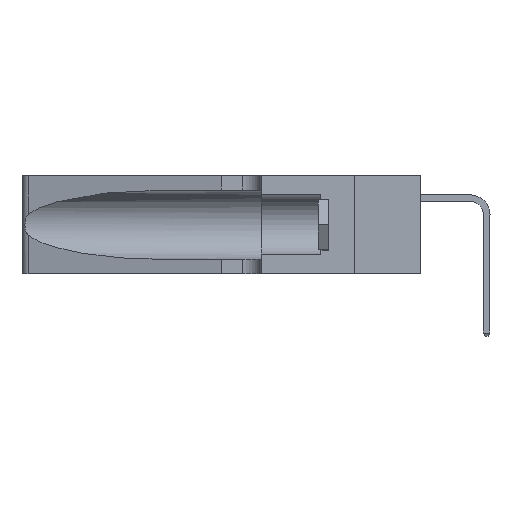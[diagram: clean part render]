
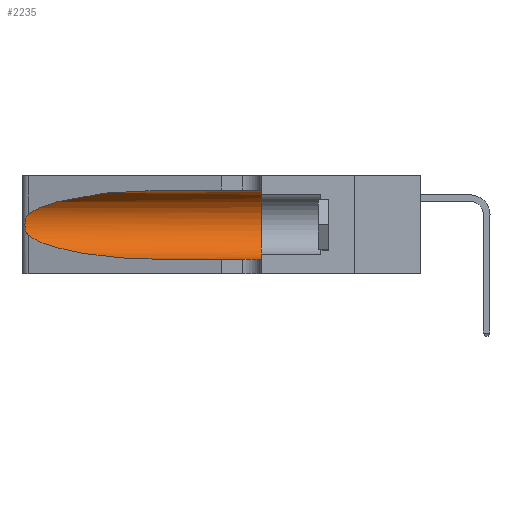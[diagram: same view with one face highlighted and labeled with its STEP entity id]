
A CAD part, left-side view. The second image highlights one B-rep face of the part: STEP entity #2235.
In plain terms, the highlighted cylindrical face has radius 3.308 mm (diameter 6.617 mm), a partial arc.
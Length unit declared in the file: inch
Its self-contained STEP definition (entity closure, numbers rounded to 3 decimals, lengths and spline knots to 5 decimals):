
#23 = ORIENTED_EDGE ( 'NONE', *, *, #29690, .T. ) ;
#699 = CARTESIAN_POINT ( 'NONE',  ( 0.25487, 1.22718, 0.22369 ) ) ;
#838 = CARTESIAN_POINT ( 'NONE',  ( 0.25487, 1.22718, 0.14631 ) ) ;
#2235 = ADVANCED_FACE ( 'NONE', ( #28565 ), #5100, .F. ) ;
#2545 = VERTEX_POINT ( 'NONE', #19586 ) ;
#2851 = CARTESIAN_POINT ( 'NONE',  ( 0.1305, 1.61858, 0.185 ) ) ;
#3192 = CARTESIAN_POINT ( 'NONE',  ( 0.1305, 0.35, 0.185 ) ) ;
#3788 = CARTESIAN_POINT ( 'NONE',  ( 0.25639, 1.23184, 0.21858 ) ) ;
#4762 = AXIS2_PLACEMENT_3D ( 'NONE', #3192, #24123, #6251 ) ;
#5100 = CYLINDRICAL_SURFACE ( 'NONE', #35761, 0.13025 ) ;
#6251 = DIRECTION ( 'NONE',  ( 0., 0., 1. ) ) ;
#6807 = VECTOR ( 'NONE', #11684, 39.37008 ) ;
#6823 = CARTESIAN_POINT ( 'NONE',  ( 0.25854, 1.2359, 0.20912 ) ) ;
#7837 = ORIENTED_EDGE ( 'NONE', *, *, #37519, .T. ) ;
#8177 = ORIENTED_EDGE ( 'NONE', *, *, #27740, .T. ) ;
#9769 = VERTEX_POINT ( 'NONE', #30126 ) ;
#9892 = CARTESIAN_POINT ( 'NONE',  ( 0.26075, 1.23896, 0.19203 ) ) ;
#10110 = CARTESIAN_POINT ( 'NONE',  ( 0.1305, 0.72297, 0.31525 ) ) ;
#10284 = VERTEX_POINT ( 'NONE', #24177 ) ;
#11684 = DIRECTION ( 'NONE',  ( 0., -1., 0. ) ) ;
#12127 = EDGE_LOOP ( 'NONE', ( #7837, #23, #37680, #8177, #34746, #33421 ) ) ;
#12278 = CIRCLE ( 'NONE', #4762, 0.13025 ) ;
#12425 = VERTEX_POINT ( 'NONE', #16951 ) ;
#12907 = CARTESIAN_POINT ( 'NONE',  ( 0.26017, 1.23833, 0.17102 ) ) ;
#13025 = CARTESIAN_POINT ( 'NONE',  ( 0.1305, 0.72297, 0.31525 ) ) ;
#14806 = LINE ( 'NONE', #26445, #6807 ) ;
#15371 =( BOUNDED_CURVE ( )  B_SPLINE_CURVE ( 3, ( #17970, #35476, #38403, #20955 ),
 .UNSPECIFIED., .F., .F. ) 
 B_SPLINE_CURVE_WITH_KNOTS ( ( 4, 4 ),
 ( 3.44316, 4.71239 ),
 .UNSPECIFIED. ) 
 CURVE ( )  GEOMETRIC_REPRESENTATION_ITEM ( )  RATIONAL_B_SPLINE_CURVE ( ( 1., 0.87, 0.87, 1. ) ) 
 REPRESENTATION_ITEM ( '' )  );
#15899 = CARTESIAN_POINT ( 'NONE',  ( 0.25789, 1.23486, 0.15765 ) ) ;
#16951 = CARTESIAN_POINT ( 'NONE',  ( 0.25487, 1.22718, 0.22369 ) ) ;
#17873 = EDGE_CURVE ( 'NONE', #23517, #10284, #33906, .T. ) ;
#17970 = CARTESIAN_POINT ( 'NONE',  ( 0.25487, 1.22718, 0.14631 ) ) ;
#18939 = CARTESIAN_POINT ( 'NONE',  ( 0.25555, 1.22993, 0.14849 ) ) ;
#19046 = CARTESIAN_POINT ( 'NONE',  ( 0.25487, 1.22718, 0.22369 ) ) ;
#19586 = CARTESIAN_POINT ( 'NONE',  ( 0.1305, 0.72297, 0.05475 ) ) ;
#20955 = CARTESIAN_POINT ( 'NONE',  ( 0.1305, 0.72297, 0.05475 ) ) ;
#21750 = CARTESIAN_POINT ( 'NONE',  ( 0.25555, 1.22994, 0.2215 ) ) ;
#23517 = VERTEX_POINT ( 'NONE', #10110 ) ;
#24123 = DIRECTION ( 'NONE',  ( 0., 1., 0. ) ) ;
#24177 = CARTESIAN_POINT ( 'NONE',  ( 0.1305, 0.35, 0.31525 ) ) ;
#24687 = CARTESIAN_POINT ( 'NONE',  ( 0.25787, 1.23484, 0.2124 ) ) ;
#26046 = CARTESIAN_POINT ( 'NONE',  ( 0.1305, 0.35, 0.05475 ) ) ;
#26445 = CARTESIAN_POINT ( 'NONE',  ( 0.1305, 1.61858, 0.05475 ) ) ;
#26879 = DIRECTION ( 'NONE',  ( 0., -1., 0. ) ) ;
#27414 =( BOUNDED_CURVE ( )  B_SPLINE_CURVE ( 3, ( #13025, #30702, #36532, #19046 ),
 .UNSPECIFIED., .F., .T. ) 
 B_SPLINE_CURVE_WITH_KNOTS ( ( 4, 4 ),
 ( 1.5708, 2.84003 ),
 .UNSPECIFIED. ) 
 CURVE ( )  GEOMETRIC_REPRESENTATION_ITEM ( )  RATIONAL_B_SPLINE_CURVE ( ( 1., 0.87, 0.87, 1. ) ) 
 REPRESENTATION_ITEM ( '' )  );
#27662 = CARTESIAN_POINT ( 'NONE',  ( 0.26018, 1.23835, 0.19895 ) ) ;
#27740 = EDGE_CURVE ( 'NONE', #2545, #33743, #14806, .T. ) ;
#27801 = EDGE_CURVE ( 'NONE', #9769, #2545, #15371, .T. ) ;
#28565 = FACE_OUTER_BOUND ( 'NONE', #12127, .T. ) ;
#29187 = DIRECTION ( 'NONE',  ( 0., -1., 0. ) ) ;
#29690 = EDGE_CURVE ( 'NONE', #12425, #9769, #34393, .T. ) ;
#29830 = DIRECTION ( 'NONE',  ( 0., 0., -1. ) ) ;
#30126 = CARTESIAN_POINT ( 'NONE',  ( 0.25487, 1.22718, 0.14631 ) ) ;
#30190 = EDGE_CURVE ( 'NONE', #10284, #33743, #12278, .T. ) ;
#30590 = CARTESIAN_POINT ( 'NONE',  ( 0.26075, 1.23896, 0.178 ) ) ;
#30702 = CARTESIAN_POINT ( 'NONE',  ( 0.18966, 0.96281, 0.31525 ) ) ;
#33000 = VECTOR ( 'NONE', #29187, 39.37008 ) ;
#33421 = ORIENTED_EDGE ( 'NONE', *, *, #17873, .F. ) ;
#33506 = CARTESIAN_POINT ( 'NONE',  ( 0.25856, 1.23593, 0.16098 ) ) ;
#33743 = VERTEX_POINT ( 'NONE', #26046 ) ;
#33906 = LINE ( 'NONE', #34894, #33000 ) ;
#34393 = B_SPLINE_CURVE_WITH_KNOTS ( 'NONE', 3,
 ( #699, #21750, #3788, #24687, #6823, #27662, #9892, #30590, #12907, #33506, #15899, #36412, #18939, #838 ),
 .UNSPECIFIED., .F., .F.,
 ( 4, 2, 2, 2, 2, 2, 4 ),
 ( 0., 0.00027, 0.00053, 0.00107, 0.0016, 0.00187, 0.00214 ),
 .UNSPECIFIED. ) ;
#34746 = ORIENTED_EDGE ( 'NONE', *, *, #30190, .F. ) ;
#34894 = CARTESIAN_POINT ( 'NONE',  ( 0.1305, 1.61858, 0.31525 ) ) ;
#35476 = CARTESIAN_POINT ( 'NONE',  ( 0.2373, 1.15595, 0.08982 ) ) ;
#35761 = AXIS2_PLACEMENT_3D ( 'NONE', #2851, #26879, #29830 ) ;
#36412 = CARTESIAN_POINT ( 'NONE',  ( 0.25639, 1.23186, 0.15144 ) ) ;
#36532 = CARTESIAN_POINT ( 'NONE',  ( 0.2373, 1.15595, 0.28018 ) ) ;
#37519 = EDGE_CURVE ( 'NONE', #23517, #12425, #27414, .T. ) ;
#37680 = ORIENTED_EDGE ( 'NONE', *, *, #27801, .T. ) ;
#38403 = CARTESIAN_POINT ( 'NONE',  ( 0.18966, 0.96281, 0.05475 ) ) ;
